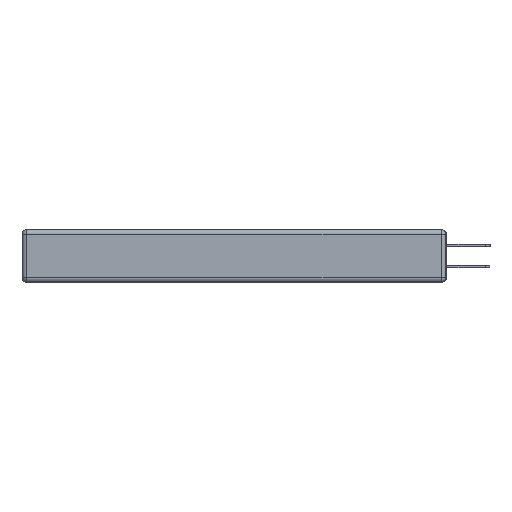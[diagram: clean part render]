
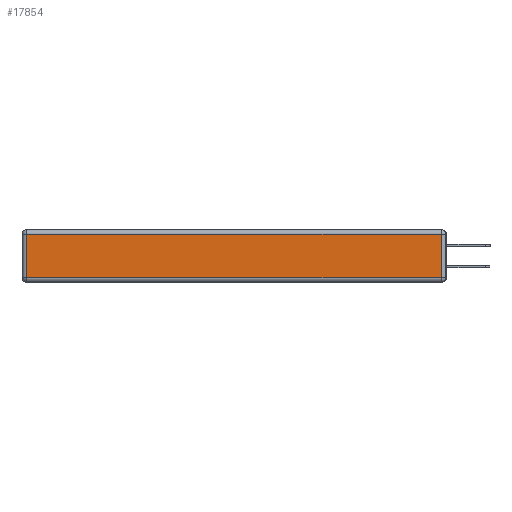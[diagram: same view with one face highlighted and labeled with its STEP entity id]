
A CAD part, left-side view. The second image highlights one B-rep face of the part: STEP entity #17854.
In plain terms, the highlighted planar face has unit normal (-1, 0, 0).
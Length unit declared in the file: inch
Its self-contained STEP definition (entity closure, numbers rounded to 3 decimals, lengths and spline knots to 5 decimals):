
#1063 = CARTESIAN_POINT ( 'NONE',  ( 0., 0.03, -0.03 ) ) ;
#1223 = ORIENTED_EDGE ( 'NONE', *, *, #19987, .T. ) ;
#1590 = LINE ( 'NONE', #6673, #5977 ) ;
#2398 = DIRECTION ( 'NONE',  ( 0., 0., -1. ) ) ;
#2929 = VERTEX_POINT ( 'NONE', #6009 ) ;
#3068 = CARTESIAN_POINT ( 'NONE',  ( 0., 0., -0.343 ) ) ;
#3085 = CARTESIAN_POINT ( 'NONE',  ( 0., 0.03, -0.343 ) ) ;
#3140 = LINE ( 'NONE', #11565, #14225 ) ;
#3141 = DIRECTION ( 'NONE',  ( -1., 0., 0. ) ) ;
#3249 = ORIENTED_EDGE ( 'NONE', *, *, #11668, .T. ) ;
#4674 = DIRECTION ( 'NONE',  ( 0., 0., 1. ) ) ;
#4766 = ORIENTED_EDGE ( 'NONE', *, *, #15225, .T. ) ;
#4841 = EDGE_CURVE ( 'NONE', #13659, #19512, #17870, .T. ) ;
#5207 = AXIS2_PLACEMENT_3D ( 'NONE', #3068, #3141, #17460 ) ;
#5977 = VECTOR ( 'NONE', #17666, 39.37008 ) ;
#6009 = CARTESIAN_POINT ( 'NONE',  ( 0., 2.72, -0.03 ) ) ;
#6130 = FACE_OUTER_BOUND ( 'NONE', #13923, .T. ) ;
#6673 = CARTESIAN_POINT ( 'NONE',  ( 0., 2.75, -0.03 ) ) ;
#7151 = CARTESIAN_POINT ( 'NONE',  ( 0., 0.03, -0.313 ) ) ;
#7302 = CARTESIAN_POINT ( 'NONE',  ( 0., 2.72, -0.313 ) ) ;
#9483 = VECTOR ( 'NONE', #4674, 39.37008 ) ;
#9911 = VECTOR ( 'NONE', #2398, 39.37008 ) ;
#9998 = ORIENTED_EDGE ( 'NONE', *, *, #4841, .T. ) ;
#11565 = CARTESIAN_POINT ( 'NONE',  ( 0., 0., -0.313 ) ) ;
#11668 = EDGE_CURVE ( 'NONE', #2929, #14560, #12628, .T. ) ;
#11906 = CARTESIAN_POINT ( 'NONE',  ( 0., 2.72, -0.343 ) ) ;
#12628 = LINE ( 'NONE', #11906, #9911 ) ;
#13659 = VERTEX_POINT ( 'NONE', #7151 ) ;
#13923 = EDGE_LOOP ( 'NONE', ( #1223, #9998, #4766, #3249 ) ) ;
#14225 = VECTOR ( 'NONE', #16321, 39.37008 ) ;
#14560 = VERTEX_POINT ( 'NONE', #7302 ) ;
#15225 = EDGE_CURVE ( 'NONE', #19512, #2929, #1590, .T. ) ;
#16321 = DIRECTION ( 'NONE',  ( 0., -1., 0. ) ) ;
#17460 = DIRECTION ( 'NONE',  ( 0., 0., 1. ) ) ;
#17666 = DIRECTION ( 'NONE',  ( 0., 1., 0. ) ) ;
#17854 = ADVANCED_FACE ( 'NONE', ( #6130 ), #20344, .T. ) ;
#17870 = LINE ( 'NONE', #3085, #9483 ) ;
#19512 = VERTEX_POINT ( 'NONE', #1063 ) ;
#19987 = EDGE_CURVE ( 'NONE', #14560, #13659, #3140, .T. ) ;
#20344 = PLANE ( 'NONE',  #5207 ) ;
